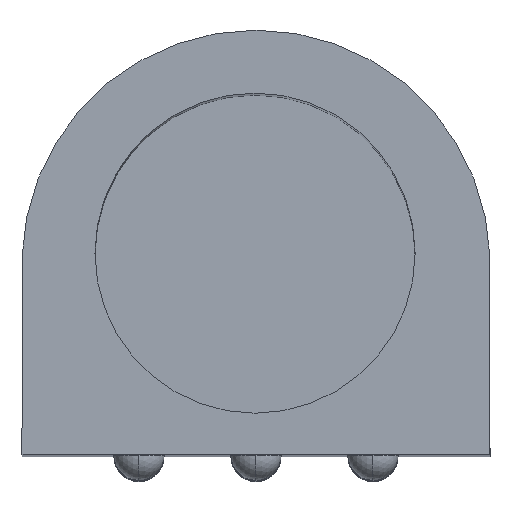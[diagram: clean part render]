
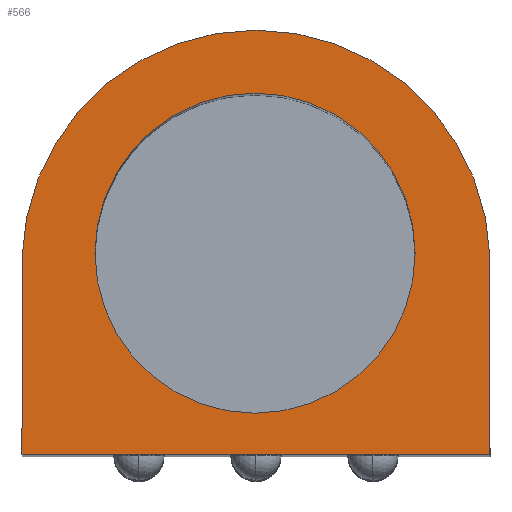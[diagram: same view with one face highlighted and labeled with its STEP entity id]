
A CAD part, top view. The second image highlights one B-rep face of the part: STEP entity #566.
In plain terms, the highlighted planar face has unit normal (0, 0, 1).
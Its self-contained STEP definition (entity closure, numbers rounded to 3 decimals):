
#46 = LINE ( 'NONE', #1047, #452 ) ;
#58 = DIRECTION ( 'NONE',  ( 0., -1., 0. ) ) ;
#70 = AXIS2_PLACEMENT_3D ( 'NONE', #934, #816, #1329 ) ;
#87 = ORIENTED_EDGE ( 'NONE', *, *, #1158, .T. ) ;
#124 = CARTESIAN_POINT ( 'NONE',  ( -63.561, 40.242, 3.642 ) ) ;
#130 = DIRECTION ( 'NONE',  ( 0., 0., 1. ) ) ;
#164 = EDGE_CURVE ( 'NONE', #1365, #636, #676, .T. ) ;
#170 = EDGE_CURVE ( 'NONE', #1088, #432, #619, .T. ) ;
#185 = VERTEX_POINT ( 'NONE', #437 ) ;
#287 = EDGE_CURVE ( 'NONE', #185, #532, #1093, .T. ) ;
#334 = FACE_OUTER_BOUND ( 'NONE', #1359, .T. ) ;
#397 = EDGE_CURVE ( 'NONE', #432, #1088, #1433, .T. ) ;
#432 = VERTEX_POINT ( 'NONE', #1042 ) ;
#437 = CARTESIAN_POINT ( 'NONE',  ( -94.752, 39.919, 3.642 ) ) ;
#452 = VECTOR ( 'NONE', #1552, 1000. ) ;
#520 = DIRECTION ( 'NONE',  ( 0., 0., 1. ) ) ;
#532 = VERTEX_POINT ( 'NONE', #825 ) ;
#566 = ADVANCED_FACE ( 'NONE', ( #334, #958 ), #839, .F. ) ;
#567 = CARTESIAN_POINT ( 'NONE',  ( -57.618, 39.919, 3.642 ) ) ;
#619 = CIRCLE ( 'NONE', #70, 12.7 ) ;
#636 = VERTEX_POINT ( 'NONE', #966 ) ;
#676 = LINE ( 'NONE', #1180, #1336 ) ;
#719 = ORIENTED_EDGE ( 'NONE', *, *, #397, .F. ) ;
#816 = DIRECTION ( 'NONE',  ( 0., 0., 1. ) ) ;
#825 = CARTESIAN_POINT ( 'NONE',  ( -94.752, 24.278, 3.642 ) ) ;
#839 = PLANE ( 'NONE',  #1461 ) ;
#848 = EDGE_CURVE ( 'NONE', #532, #636, #46, .T. ) ;
#892 = EDGE_LOOP ( 'NONE', ( #1378, #719 ) ) ;
#932 = ORIENTED_EDGE ( 'NONE', *, *, #848, .T. ) ;
#934 = CARTESIAN_POINT ( 'NONE',  ( -76.261, 40.242, 3.642 ) ) ;
#949 = ORIENTED_EDGE ( 'NONE', *, *, #164, .F. ) ;
#950 = DIRECTION ( 'NONE',  ( 0., 0., -1. ) ) ;
#958 = FACE_BOUND ( 'NONE', #892, .T. ) ;
#966 = CARTESIAN_POINT ( 'NONE',  ( -57.618, 24.278, 3.642 ) ) ;
#1008 = DIRECTION ( 'NONE',  ( 1., 0., 0. ) ) ;
#1023 = AXIS2_PLACEMENT_3D ( 'NONE', #1156, #520, #1008 ) ;
#1029 = CARTESIAN_POINT ( 'NONE',  ( -76.261, 40.242, 3.642 ) ) ;
#1042 = CARTESIAN_POINT ( 'NONE',  ( -88.961, 40.242, 3.642 ) ) ;
#1047 = CARTESIAN_POINT ( 'NONE',  ( -94.752, 24.278, 3.642 ) ) ;
#1087 = VECTOR ( 'NONE', #1221, 1000. ) ;
#1088 = VERTEX_POINT ( 'NONE', #124 ) ;
#1093 = LINE ( 'NONE', #1243, #1087 ) ;
#1156 = CARTESIAN_POINT ( 'NONE',  ( -76.185, 39.361, 3.642 ) ) ;
#1158 = EDGE_CURVE ( 'NONE', #1365, #185, #1187, .T. ) ;
#1161 = DIRECTION ( 'NONE',  ( 1., 0., 0. ) ) ;
#1180 = CARTESIAN_POINT ( 'NONE',  ( -57.618, 39.919, 3.642 ) ) ;
#1187 = CIRCLE ( 'NONE', #1023, 18.575 ) ;
#1198 = ORIENTED_EDGE ( 'NONE', *, *, #287, .T. ) ;
#1221 = DIRECTION ( 'NONE',  ( 0., -1., 0. ) ) ;
#1243 = CARTESIAN_POINT ( 'NONE',  ( -94.752, 39.919, 3.642 ) ) ;
#1318 = DIRECTION ( 'NONE',  ( -1., 0., 0. ) ) ;
#1329 = DIRECTION ( 'NONE',  ( 1., 0., 0. ) ) ;
#1331 = AXIS2_PLACEMENT_3D ( 'NONE', #1029, #130, #1161 ) ;
#1336 = VECTOR ( 'NONE', #58, 1000. ) ;
#1359 = EDGE_LOOP ( 'NONE', ( #949, #87, #1198, #932 ) ) ;
#1365 = VERTEX_POINT ( 'NONE', #567 ) ;
#1378 = ORIENTED_EDGE ( 'NONE', *, *, #170, .F. ) ;
#1433 = CIRCLE ( 'NONE', #1331, 12.7 ) ;
#1461 = AXIS2_PLACEMENT_3D ( 'NONE', #1587, #950, #1318 ) ;
#1552 = DIRECTION ( 'NONE',  ( 1., 0., 0. ) ) ;
#1587 = CARTESIAN_POINT ( 'NONE',  ( -395.136, -37.369, 3.642 ) ) ;
